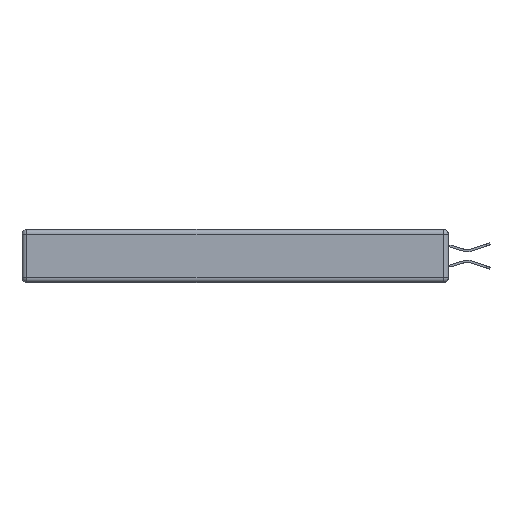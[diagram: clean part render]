
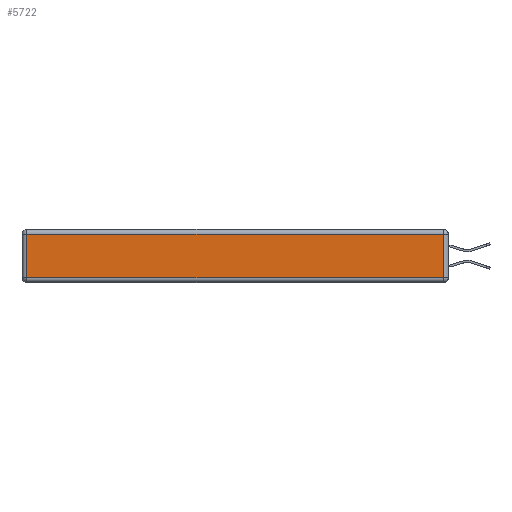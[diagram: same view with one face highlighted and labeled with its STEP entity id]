
A CAD part, left-side view. The second image highlights one B-rep face of the part: STEP entity #5722.
In plain terms, the highlighted planar face has unit normal (-1, 0, 0).
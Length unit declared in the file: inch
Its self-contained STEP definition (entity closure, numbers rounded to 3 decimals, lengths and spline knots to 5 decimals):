
#2118 = VERTEX_POINT ( 'NONE', #5725 ) ;
#2167 = LINE ( 'NONE', #7404, #2408 ) ;
#2408 = VECTOR ( 'NONE', #3113, 39.37008 ) ;
#2809 = CARTESIAN_POINT ( 'NONE',  ( 0., 2.75, -0.03 ) ) ;
#2859 = AXIS2_PLACEMENT_3D ( 'NONE', #8686, #7342, #16157 ) ;
#2907 = CARTESIAN_POINT ( 'NONE',  ( 0., 0.03, -0.313 ) ) ;
#3113 = DIRECTION ( 'NONE',  ( 0., -1., 0. ) ) ;
#3516 = FACE_OUTER_BOUND ( 'NONE', #9242, .T. ) ;
#5722 = ADVANCED_FACE ( 'NONE', ( #3516 ), #13136, .T. ) ;
#5725 = CARTESIAN_POINT ( 'NONE',  ( 0., 2.72, -0.313 ) ) ;
#5733 = VERTEX_POINT ( 'NONE', #2907 ) ;
#6332 = ORIENTED_EDGE ( 'NONE', *, *, #18459, .T. ) ;
#6707 = CARTESIAN_POINT ( 'NONE',  ( 0., 2.72, -0.03 ) ) ;
#7342 = DIRECTION ( 'NONE',  ( -1., 0., 0. ) ) ;
#7404 = CARTESIAN_POINT ( 'NONE',  ( 0., 0., -0.313 ) ) ;
#8292 = CARTESIAN_POINT ( 'NONE',  ( 0., 2.72, -0.343 ) ) ;
#8435 = LINE ( 'NONE', #17951, #16022 ) ;
#8686 = CARTESIAN_POINT ( 'NONE',  ( 0., 0., -0.343 ) ) ;
#9009 = CARTESIAN_POINT ( 'NONE',  ( 0., 0.03, -0.03 ) ) ;
#9236 = EDGE_CURVE ( 'NONE', #17270, #2118, #13866, .T. ) ;
#9242 = EDGE_LOOP ( 'NONE', ( #6332, #12314, #18530, #9846 ) ) ;
#9787 = DIRECTION ( 'NONE',  ( 0., 0., -1. ) ) ;
#9846 = ORIENTED_EDGE ( 'NONE', *, *, #9236, .T. ) ;
#10043 = VECTOR ( 'NONE', #10148, 39.37008 ) ;
#10148 = DIRECTION ( 'NONE',  ( 0., 1., 0. ) ) ;
#12314 = ORIENTED_EDGE ( 'NONE', *, *, #17631, .T. ) ;
#13136 = PLANE ( 'NONE',  #2859 ) ;
#13866 = LINE ( 'NONE', #8292, #17767 ) ;
#13964 = LINE ( 'NONE', #2809, #10043 ) ;
#16022 = VECTOR ( 'NONE', #16849, 39.37008 ) ;
#16157 = DIRECTION ( 'NONE',  ( 0., 0., 1. ) ) ;
#16849 = DIRECTION ( 'NONE',  ( 0., 0., 1. ) ) ;
#17270 = VERTEX_POINT ( 'NONE', #6707 ) ;
#17631 = EDGE_CURVE ( 'NONE', #5733, #17639, #8435, .T. ) ;
#17639 = VERTEX_POINT ( 'NONE', #9009 ) ;
#17767 = VECTOR ( 'NONE', #9787, 39.37008 ) ;
#17842 = EDGE_CURVE ( 'NONE', #17639, #17270, #13964, .T. ) ;
#17951 = CARTESIAN_POINT ( 'NONE',  ( 0., 0.03, -0.343 ) ) ;
#18459 = EDGE_CURVE ( 'NONE', #2118, #5733, #2167, .T. ) ;
#18530 = ORIENTED_EDGE ( 'NONE', *, *, #17842, .T. ) ;
